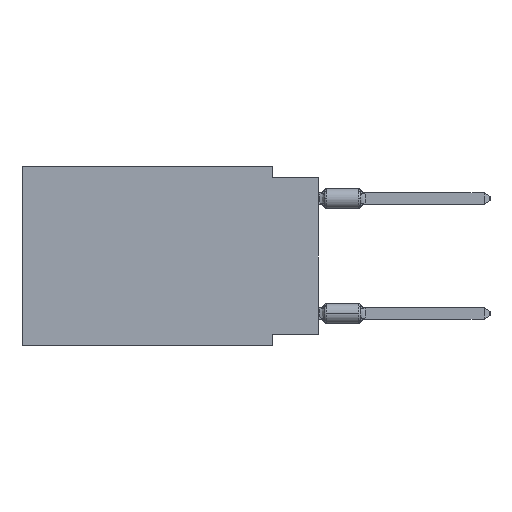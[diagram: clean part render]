
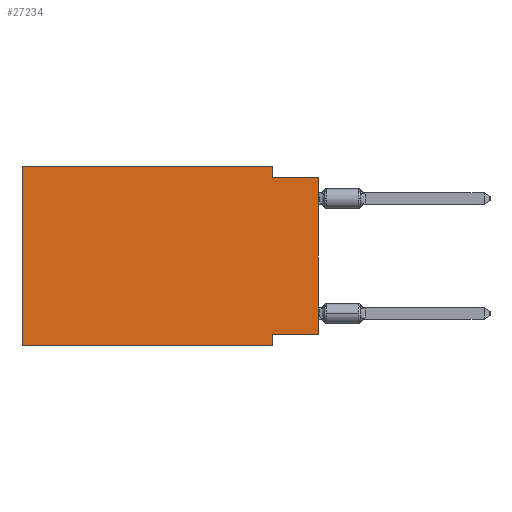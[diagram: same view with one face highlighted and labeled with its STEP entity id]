
A CAD part, left-side view. The second image highlights one B-rep face of the part: STEP entity #27234.
In plain terms, the highlighted planar face has unit normal (-1, 0, 0).
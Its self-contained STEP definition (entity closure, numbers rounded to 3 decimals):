
#182 = EDGE_CURVE ( 'NONE', #34745, #13775, #37341, .T. ) ;
#1861 = ORIENTED_EDGE ( 'NONE', *, *, #33776, .F. ) ;
#1924 = VERTEX_POINT ( 'NONE', #18432 ) ;
#2703 = DIRECTION ( 'NONE',  ( 0., 1., 0. ) ) ;
#3212 = VECTOR ( 'NONE', #2703, 1000. ) ;
#3722 = LINE ( 'NONE', #4140, #34072 ) ;
#3932 = DIRECTION ( 'NONE',  ( 0., 0., -1. ) ) ;
#4140 = CARTESIAN_POINT ( 'NONE',  ( 0., 2.54, 0. ) ) ;
#4276 = DIRECTION ( 'NONE',  ( 0., 0., -1. ) ) ;
#5908 = LINE ( 'NONE', #27889, #38157 ) ;
#6019 = LINE ( 'NONE', #31119, #3212 ) ;
#6102 = VECTOR ( 'NONE', #10236, 1000. ) ;
#7581 = ORIENTED_EDGE ( 'NONE', *, *, #13626, .F. ) ;
#7836 = LINE ( 'NONE', #20278, #13043 ) ;
#8122 = EDGE_CURVE ( 'NONE', #32169, #21081, #5908, .T. ) ;
#8316 = DIRECTION ( 'NONE',  ( 0., 0., 1. ) ) ;
#8612 = DIRECTION ( 'NONE',  ( 0., -1., 0. ) ) ;
#9316 = CARTESIAN_POINT ( 'NONE',  ( 0., 2.54, -9.271 ) ) ;
#10236 = DIRECTION ( 'NONE',  ( 0., 0., -1. ) ) ;
#10256 = DIRECTION ( 'NONE',  ( 0., -1., 0. ) ) ;
#10333 = ORIENTED_EDGE ( 'NONE', *, *, #28219, .F. ) ;
#11421 = EDGE_CURVE ( 'NONE', #17585, #32681, #7836, .T. ) ;
#11546 = ORIENTED_EDGE ( 'NONE', *, *, #11421, .F. ) ;
#11905 = CARTESIAN_POINT ( 'NONE',  ( 0., 2.54, 0. ) ) ;
#11962 = AXIS2_PLACEMENT_3D ( 'NONE', #13995, #35593, #4276 ) ;
#12928 = CARTESIAN_POINT ( 'NONE',  ( 0., 16.383, 0. ) ) ;
#13043 = VECTOR ( 'NONE', #29432, 1000. ) ;
#13391 = FACE_OUTER_BOUND ( 'NONE', #13655, .T. ) ;
#13626 = EDGE_CURVE ( 'NONE', #1924, #13775, #16479, .T. ) ;
#13655 = EDGE_LOOP ( 'NONE', ( #23598, #7581, #1861, #11546, #10333, #34953, #33742, #39777 ) ) ;
#13775 = VERTEX_POINT ( 'NONE', #34020 ) ;
#13995 = CARTESIAN_POINT ( 'NONE',  ( 0., 16.383, 0. ) ) ;
#15437 = VECTOR ( 'NONE', #8316, 1000. ) ;
#16479 = LINE ( 'NONE', #38674, #25761 ) ;
#16974 = CARTESIAN_POINT ( 'NONE',  ( 0., 16.383, -9.906 ) ) ;
#17553 = EDGE_CURVE ( 'NONE', #33707, #21081, #37829, .T. ) ;
#17585 = VERTEX_POINT ( 'NONE', #12928 ) ;
#18432 = CARTESIAN_POINT ( 'NONE',  ( 0., 2.54, -0.635 ) ) ;
#19007 = LINE ( 'NONE', #32279, #26475 ) ;
#20278 = CARTESIAN_POINT ( 'NONE',  ( 0., 16.383, 0. ) ) ;
#21081 = VERTEX_POINT ( 'NONE', #24133 ) ;
#22937 = PLANE ( 'NONE',  #11962 ) ;
#23598 = ORIENTED_EDGE ( 'NONE', *, *, #182, .T. ) ;
#24133 = CARTESIAN_POINT ( 'NONE',  ( 0., 2.54, -9.906 ) ) ;
#25761 = VECTOR ( 'NONE', #10256, 1000. ) ;
#26475 = VECTOR ( 'NONE', #40991, 1000. ) ;
#27234 = ADVANCED_FACE ( 'NONE', ( #13391 ), #22937, .F. ) ;
#27889 = CARTESIAN_POINT ( 'NONE',  ( 0., 16.383, -9.906 ) ) ;
#28219 = EDGE_CURVE ( 'NONE', #32169, #17585, #19007, .T. ) ;
#29432 = DIRECTION ( 'NONE',  ( 0., -1., 0. ) ) ;
#31119 = CARTESIAN_POINT ( 'NONE',  ( 0., 0., -9.271 ) ) ;
#32169 = VERTEX_POINT ( 'NONE', #16974 ) ;
#32279 = CARTESIAN_POINT ( 'NONE',  ( 0., 16.383, 0. ) ) ;
#32681 = VERTEX_POINT ( 'NONE', #11905 ) ;
#33707 = VERTEX_POINT ( 'NONE', #9316 ) ;
#33742 = ORIENTED_EDGE ( 'NONE', *, *, #17553, .F. ) ;
#33776 = EDGE_CURVE ( 'NONE', #32681, #1924, #3722, .T. ) ;
#34020 = CARTESIAN_POINT ( 'NONE',  ( 0., 0., -0.635 ) ) ;
#34072 = VECTOR ( 'NONE', #3932, 1000. ) ;
#34745 = VERTEX_POINT ( 'NONE', #38757 ) ;
#34953 = ORIENTED_EDGE ( 'NONE', *, *, #8122, .T. ) ;
#35593 = DIRECTION ( 'NONE',  ( 1., 0., 0. ) ) ;
#36724 = CARTESIAN_POINT ( 'NONE',  ( 0., 0., 0. ) ) ;
#37341 = LINE ( 'NONE', #36724, #15437 ) ;
#37453 = EDGE_CURVE ( 'NONE', #34745, #33707, #6019, .T. ) ;
#37829 = LINE ( 'NONE', #38655, #6102 ) ;
#38157 = VECTOR ( 'NONE', #8612, 1000. ) ;
#38655 = CARTESIAN_POINT ( 'NONE',  ( 0., 2.54, -9.906 ) ) ;
#38674 = CARTESIAN_POINT ( 'NONE',  ( 0., 0., -0.635 ) ) ;
#38757 = CARTESIAN_POINT ( 'NONE',  ( 0., 0., -9.271 ) ) ;
#39777 = ORIENTED_EDGE ( 'NONE', *, *, #37453, .F. ) ;
#40991 = DIRECTION ( 'NONE',  ( 0., 0., 1. ) ) ;
